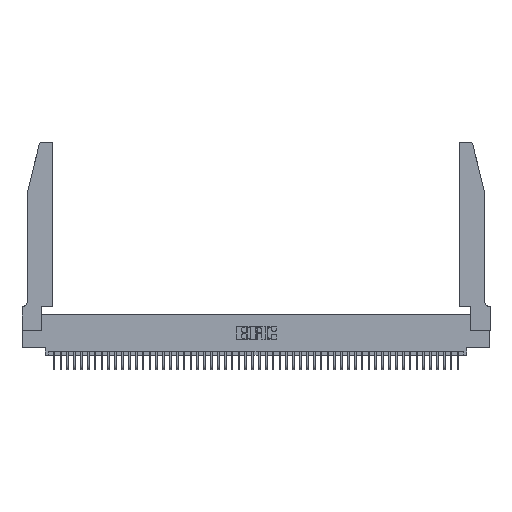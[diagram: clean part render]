
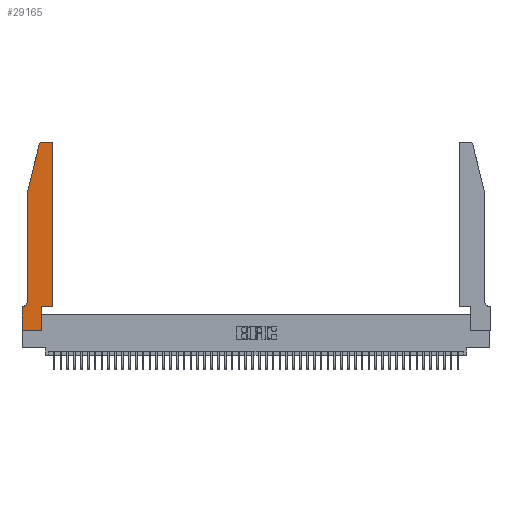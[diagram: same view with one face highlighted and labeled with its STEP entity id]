
A CAD part, top view. The second image highlights one B-rep face of the part: STEP entity #29165.
In plain terms, the highlighted planar face has unit normal (0, 0, 1).
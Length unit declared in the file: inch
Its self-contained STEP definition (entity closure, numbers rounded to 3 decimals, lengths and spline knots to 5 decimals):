
#35 = LINE ( 'NONE', #47200, #39719 ) ;
#447 = ORIENTED_EDGE ( 'NONE', *, *, #13025, .T. ) ;
#565 = LINE ( 'NONE', #49147, #49495 ) ;
#623 = CARTESIAN_POINT ( 'NONE',  ( 0.284, 2.75, 0.37 ) ) ;
#900 = CARTESIAN_POINT ( 'NONE',  ( 0.2865, 0., 0.37 ) ) ;
#1923 = CARTESIAN_POINT ( 'NONE',  ( 0., 0.35, 0.37 ) ) ;
#2225 = EDGE_LOOP ( 'NONE', ( #20807, #35230, #14241, #23005, #31696, #18669, #28369, #447, #13478, #38011, #12507, #45868 ) ) ;
#2549 = VECTOR ( 'NONE', #16534, 39.37008 ) ;
#2996 = CARTESIAN_POINT ( 'NONE',  ( 0.0755, 0.42, 0.37 ) ) ;
#3159 = DIRECTION ( 'NONE',  ( -1., 0., 0. ) ) ;
#4299 = CIRCLE ( 'NONE', #23302, 0.03 ) ;
#4465 = LINE ( 'NONE', #4594, #45413 ) ;
#4594 = CARTESIAN_POINT ( 'NONE',  ( 0.0755, 2., 0.37 ) ) ;
#4780 = LINE ( 'NONE', #50597, #35214 ) ;
#5043 = CARTESIAN_POINT ( 'NONE',  ( 0., 0.35, 0.37 ) ) ;
#5286 = VERTEX_POINT ( 'NONE', #623 ) ;
#5420 = DIRECTION ( 'NONE',  ( 0., 0., 1. ) ) ;
#5425 = VERTEX_POINT ( 'NONE', #5458 ) ;
#5458 = CARTESIAN_POINT ( 'NONE',  ( 0., 0., 0.37 ) ) ;
#6047 = VECTOR ( 'NONE', #31931, 39.37008 ) ;
#6608 = CARTESIAN_POINT ( 'NONE',  ( 0.4205, 2.75, 0.37 ) ) ;
#7365 = VECTOR ( 'NONE', #13429, 39.37008 ) ;
#10936 = VERTEX_POINT ( 'NONE', #31539 ) ;
#11749 = CARTESIAN_POINT ( 'NONE',  ( 0., 0., 0.37 ) ) ;
#12154 = CARTESIAN_POINT ( 'NONE',  ( 0.4505, 0.35, 0.37 ) ) ;
#12507 = ORIENTED_EDGE ( 'NONE', *, *, #15587, .T. ) ;
#13025 = EDGE_CURVE ( 'NONE', #5425, #48902, #27138, .T. ) ;
#13429 = DIRECTION ( 'NONE',  ( 0., 1., 0. ) ) ;
#13478 = ORIENTED_EDGE ( 'NONE', *, *, #23878, .T. ) ;
#13485 = AXIS2_PLACEMENT_3D ( 'NONE', #16618, #44258, #20660 ) ;
#13497 = VERTEX_POINT ( 'NONE', #6608 ) ;
#13662 = EDGE_CURVE ( 'NONE', #13497, #5286, #41871, .T. ) ;
#13821 = VERTEX_POINT ( 'NONE', #28301 ) ;
#14241 = ORIENTED_EDGE ( 'NONE', *, *, #45080, .T. ) ;
#15587 = EDGE_CURVE ( 'NONE', #13821, #43132, #34228, .T. ) ;
#16534 = DIRECTION ( 'NONE',  ( 0., 1., 0. ) ) ;
#16558 = VECTOR ( 'NONE', #31532, 39.37008 ) ;
#16618 = CARTESIAN_POINT ( 'NONE',  ( 0.0055, 0.42, 0.37 ) ) ;
#17998 = PLANE ( 'NONE',  #45916 ) ;
#18669 = ORIENTED_EDGE ( 'NONE', *, *, #46709, .T. ) ;
#18912 = EDGE_CURVE ( 'NONE', #46703, #10936, #30101, .T. ) ;
#20505 = DIRECTION ( 'NONE',  ( 0., -1., 0. ) ) ;
#20618 = DIRECTION ( 'NONE',  ( 0., 0., 1. ) ) ;
#20660 = DIRECTION ( 'NONE',  ( -1., 0., 0. ) ) ;
#20807 = ORIENTED_EDGE ( 'NONE', *, *, #13662, .T. ) ;
#22003 = DIRECTION ( 'NONE',  ( 1., 0., 0. ) ) ;
#23005 = ORIENTED_EDGE ( 'NONE', *, *, #30280, .T. ) ;
#23302 = AXIS2_PLACEMENT_3D ( 'NONE', #44213, #20618, #48166 ) ;
#23878 = EDGE_CURVE ( 'NONE', #48902, #41197, #37758, .T. ) ;
#24002 = VERTEX_POINT ( 'NONE', #30582 ) ;
#24280 = EDGE_CURVE ( 'NONE', #41197, #13821, #37713, .T. ) ;
#27138 = LINE ( 'NONE', #11749, #16558 ) ;
#27374 = CIRCLE ( 'NONE', #30756, 0.03 ) ;
#28301 = CARTESIAN_POINT ( 'NONE',  ( 0.4505, 0.35, 0.37 ) ) ;
#28369 = ORIENTED_EDGE ( 'NONE', *, *, #29790, .T. ) ;
#29165 = ADVANCED_FACE ( 'NONE', ( #37239 ), #17998, .T. ) ;
#29225 = CARTESIAN_POINT ( 'NONE',  ( 0.284, 2.72, 0.37 ) ) ;
#29790 = EDGE_CURVE ( 'NONE', #36769, #5425, #565, .T. ) ;
#30101 = CIRCLE ( 'NONE', #13485, 0.07 ) ;
#30120 = VECTOR ( 'NONE', #31433, 39.37008 ) ;
#30280 = EDGE_CURVE ( 'NONE', #34698, #46703, #4465, .T. ) ;
#30582 = CARTESIAN_POINT ( 'NONE',  ( 0.25487, 2.72718, 0.37 ) ) ;
#30756 = AXIS2_PLACEMENT_3D ( 'NONE', #29225, #5420, #33196 ) ;
#31433 = DIRECTION ( 'NONE',  ( -1., 0., 0. ) ) ;
#31532 = DIRECTION ( 'NONE',  ( 1., 0., 0. ) ) ;
#31539 = CARTESIAN_POINT ( 'NONE',  ( 0.0055, 0.35, 0.37 ) ) ;
#31696 = ORIENTED_EDGE ( 'NONE', *, *, #18912, .T. ) ;
#31931 = DIRECTION ( 'NONE',  ( 1., 0., 0. ) ) ;
#32286 = CARTESIAN_POINT ( 'NONE',  ( 0.4505, 0.35, 0.37 ) ) ;
#33196 = DIRECTION ( 'NONE',  ( 1., 0., 0. ) ) ;
#34228 = LINE ( 'NONE', #32286, #2549 ) ;
#34698 = VERTEX_POINT ( 'NONE', #44862 ) ;
#35214 = VECTOR ( 'NONE', #3159, 39.37008 ) ;
#35230 = ORIENTED_EDGE ( 'NONE', *, *, #45349, .T. ) ;
#36769 = VERTEX_POINT ( 'NONE', #5043 ) ;
#37239 = FACE_OUTER_BOUND ( 'NONE', #2225, .T. ) ;
#37713 = LINE ( 'NONE', #12154, #6047 ) ;
#37758 = LINE ( 'NONE', #49031, #7365 ) ;
#38011 = ORIENTED_EDGE ( 'NONE', *, *, #24280, .T. ) ;
#38150 = CARTESIAN_POINT ( 'NONE',  ( 0.2865, 0.35, 0.37 ) ) ;
#38372 = EDGE_CURVE ( 'NONE', #43132, #13497, #4299, .T. ) ;
#39719 = VECTOR ( 'NONE', #43244, 39.37008 ) ;
#41197 = VERTEX_POINT ( 'NONE', #38150 ) ;
#41406 = DIRECTION ( 'NONE',  ( 0., -1., 0. ) ) ;
#41871 = LINE ( 'NONE', #43330, #30120 ) ;
#43132 = VERTEX_POINT ( 'NONE', #45921 ) ;
#43244 = DIRECTION ( 'NONE',  ( -0.239, -0.971, 0. ) ) ;
#43330 = CARTESIAN_POINT ( 'NONE',  ( 0.2605, 2.75, 0.37 ) ) ;
#44213 = CARTESIAN_POINT ( 'NONE',  ( 0.4205, 2.72, 0.37 ) ) ;
#44258 = DIRECTION ( 'NONE',  ( 0., 0., -1. ) ) ;
#44862 = CARTESIAN_POINT ( 'NONE',  ( 0.0755, 2., 0.37 ) ) ;
#45080 = EDGE_CURVE ( 'NONE', #24002, #34698, #35, .T. ) ;
#45349 = EDGE_CURVE ( 'NONE', #5286, #24002, #27374, .T. ) ;
#45413 = VECTOR ( 'NONE', #20505, 39.37008 ) ;
#45611 = DIRECTION ( 'NONE',  ( 0., 0., 1. ) ) ;
#45868 = ORIENTED_EDGE ( 'NONE', *, *, #38372, .T. ) ;
#45916 = AXIS2_PLACEMENT_3D ( 'NONE', #1923, #45611, #22003 ) ;
#45921 = CARTESIAN_POINT ( 'NONE',  ( 0.4505, 2.72, 0.37 ) ) ;
#46703 = VERTEX_POINT ( 'NONE', #2996 ) ;
#46709 = EDGE_CURVE ( 'NONE', #10936, #36769, #4780, .T. ) ;
#47200 = CARTESIAN_POINT ( 'NONE',  ( 0.0755, 2., 0.37 ) ) ;
#48166 = DIRECTION ( 'NONE',  ( 1., 0., 0. ) ) ;
#48902 = VERTEX_POINT ( 'NONE', #900 ) ;
#49031 = CARTESIAN_POINT ( 'NONE',  ( 0.2865, 0.35, 0.37 ) ) ;
#49147 = CARTESIAN_POINT ( 'NONE',  ( 0., 0., 0.37 ) ) ;
#49495 = VECTOR ( 'NONE', #41406, 39.37008 ) ;
#50597 = CARTESIAN_POINT ( 'NONE',  ( 0.0755, 0.35, 0.37 ) ) ;
